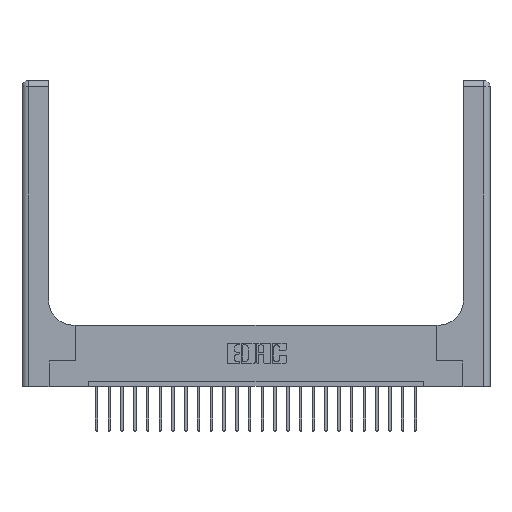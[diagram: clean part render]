
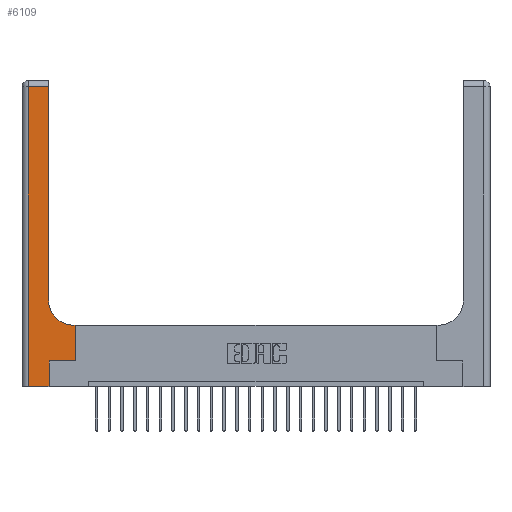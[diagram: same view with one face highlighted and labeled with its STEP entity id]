
A CAD part, top view. The second image highlights one B-rep face of the part: STEP entity #6109.
In plain terms, the highlighted planar face has unit normal (0, 0, 1).
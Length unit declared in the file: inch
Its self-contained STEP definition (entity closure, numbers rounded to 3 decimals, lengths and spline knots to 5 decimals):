
#52 = CIRCLE ( 'NONE', #3947, 0.25 ) ;
#340 = CARTESIAN_POINT ( 'NONE',  ( 0.528, 0.25, 0.37 ) ) ;
#848 = DIRECTION ( 'NONE',  ( 1., 0., 0. ) ) ;
#1018 = VERTEX_POINT ( 'NONE', #1025 ) ;
#1025 = CARTESIAN_POINT ( 'NONE',  ( 0.265, 0., 0.37 ) ) ;
#1328 = EDGE_CURVE ( 'NONE', #9289, #3444, #2215, .T. ) ;
#1359 = VECTOR ( 'NONE', #3113, 39.37008 ) ;
#1477 = VERTEX_POINT ( 'NONE', #10453 ) ;
#2215 = LINE ( 'NONE', #15375, #22464 ) ;
#2717 = VERTEX_POINT ( 'NONE', #5600 ) ;
#3113 = DIRECTION ( 'NONE',  ( 0., -1., 0. ) ) ;
#3294 = ORIENTED_EDGE ( 'NONE', *, *, #9906, .T. ) ;
#3345 = DIRECTION ( 'NONE',  ( -1., 0., 0. ) ) ;
#3418 = CARTESIAN_POINT ( 'NONE',  ( 0.06, 2.94, 0.37 ) ) ;
#3444 = VERTEX_POINT ( 'NONE', #21826 ) ;
#3483 = LINE ( 'NONE', #20137, #4670 ) ;
#3690 = PLANE ( 'NONE',  #15995 ) ;
#3947 = AXIS2_PLACEMENT_3D ( 'NONE', #6186, #13545, #848 ) ;
#4412 = CARTESIAN_POINT ( 'NONE',  ( 0.26, 2.94, 0.37 ) ) ;
#4670 = VECTOR ( 'NONE', #7568, 39.37008 ) ;
#4960 = VECTOR ( 'NONE', #17511, 39.37008 ) ;
#5282 = CARTESIAN_POINT ( 'NONE',  ( 0.26, 0.85, 0.37 ) ) ;
#5522 = FACE_OUTER_BOUND ( 'NONE', #9413, .T. ) ;
#5600 = CARTESIAN_POINT ( 'NONE',  ( 0.265, 0.25, 0.37 ) ) ;
#5604 = EDGE_CURVE ( 'NONE', #15271, #12228, #52, .T. ) ;
#5982 = EDGE_CURVE ( 'NONE', #8473, #22830, #23167, .T. ) ;
#6024 = LINE ( 'NONE', #18813, #21729 ) ;
#6109 = ADVANCED_FACE ( 'NONE', ( #5522 ), #3690, .F. ) ;
#6186 = CARTESIAN_POINT ( 'NONE',  ( 0.51, 0.85, 0.37 ) ) ;
#6567 = ORIENTED_EDGE ( 'NONE', *, *, #5604, .T. ) ;
#7208 = DIRECTION ( 'NONE',  ( 0., 0., -1. ) ) ;
#7568 = DIRECTION ( 'NONE',  ( 0., 1., 0. ) ) ;
#7877 = EDGE_CURVE ( 'NONE', #22830, #1477, #8441, .T. ) ;
#8441 = LINE ( 'NONE', #15902, #1359 ) ;
#8473 = VERTEX_POINT ( 'NONE', #4412 ) ;
#9289 = VERTEX_POINT ( 'NONE', #340 ) ;
#9413 = EDGE_LOOP ( 'NONE', ( #13953, #13611, #21633, #13463, #9802, #12706, #10533, #3294, #6567 ) ) ;
#9802 = ORIENTED_EDGE ( 'NONE', *, *, #14619, .T. ) ;
#9906 = EDGE_CURVE ( 'NONE', #3444, #15271, #18540, .T. ) ;
#10000 = CARTESIAN_POINT ( 'NONE',  ( 0., 2.94, 0.37 ) ) ;
#10453 = CARTESIAN_POINT ( 'NONE',  ( 0.06, 0., 0.37 ) ) ;
#10533 = ORIENTED_EDGE ( 'NONE', *, *, #1328, .T. ) ;
#10840 = EDGE_CURVE ( 'NONE', #2717, #9289, #6024, .T. ) ;
#11430 = EDGE_CURVE ( 'NONE', #12228, #8473, #16705, .T. ) ;
#12228 = VERTEX_POINT ( 'NONE', #5282 ) ;
#12652 = CARTESIAN_POINT ( 'NONE',  ( 0.26, 0.6, 0.37 ) ) ;
#12706 = ORIENTED_EDGE ( 'NONE', *, *, #10840, .T. ) ;
#12783 = VECTOR ( 'NONE', #20006, 39.37008 ) ;
#12957 = EDGE_CURVE ( 'NONE', #1477, #1018, #19080, .T. ) ;
#13423 = CARTESIAN_POINT ( 'NONE',  ( 0., 0., 0.37 ) ) ;
#13463 = ORIENTED_EDGE ( 'NONE', *, *, #12957, .T. ) ;
#13545 = DIRECTION ( 'NONE',  ( 0., 0., -1. ) ) ;
#13611 = ORIENTED_EDGE ( 'NONE', *, *, #5982, .T. ) ;
#13825 = CARTESIAN_POINT ( 'NONE',  ( 0.51, 0.6, 0.37 ) ) ;
#13953 = ORIENTED_EDGE ( 'NONE', *, *, #11430, .T. ) ;
#14053 = VECTOR ( 'NONE', #20971, 39.37008 ) ;
#14619 = EDGE_CURVE ( 'NONE', #1018, #2717, #3483, .T. ) ;
#15175 = DIRECTION ( 'NONE',  ( 1., 0., 0. ) ) ;
#15246 = DIRECTION ( 'NONE',  ( 0., 1., 0. ) ) ;
#15271 = VERTEX_POINT ( 'NONE', #13825 ) ;
#15375 = CARTESIAN_POINT ( 'NONE',  ( 0.528, 0.25, 0.37 ) ) ;
#15902 = CARTESIAN_POINT ( 'NONE',  ( 0.06, 3., 0.37 ) ) ;
#15995 = AXIS2_PLACEMENT_3D ( 'NONE', #21950, #7208, #3345 ) ;
#16705 = LINE ( 'NONE', #18158, #20595 ) ;
#17511 = DIRECTION ( 'NONE',  ( 1., 0., 0. ) ) ;
#18158 = CARTESIAN_POINT ( 'NONE',  ( 0.26, 3., 0.37 ) ) ;
#18540 = LINE ( 'NONE', #12652, #12783 ) ;
#18813 = CARTESIAN_POINT ( 'NONE',  ( 0.265, 0.25, 0.37 ) ) ;
#19080 = LINE ( 'NONE', #13423, #4960 ) ;
#20006 = DIRECTION ( 'NONE',  ( -1., 0., 0. ) ) ;
#20137 = CARTESIAN_POINT ( 'NONE',  ( 0.265, 0., 0.37 ) ) ;
#20334 = DIRECTION ( 'NONE',  ( 0., 1., 0. ) ) ;
#20595 = VECTOR ( 'NONE', #20334, 39.37008 ) ;
#20971 = DIRECTION ( 'NONE',  ( -1., 0., 0. ) ) ;
#21633 = ORIENTED_EDGE ( 'NONE', *, *, #7877, .T. ) ;
#21729 = VECTOR ( 'NONE', #15175, 39.37008 ) ;
#21826 = CARTESIAN_POINT ( 'NONE',  ( 0.528, 0.6, 0.37 ) ) ;
#21950 = CARTESIAN_POINT ( 'NONE',  ( 0., 3., 0.37 ) ) ;
#22464 = VECTOR ( 'NONE', #15246, 39.37008 ) ;
#22830 = VERTEX_POINT ( 'NONE', #3418 ) ;
#23167 = LINE ( 'NONE', #10000, #14053 ) ;
